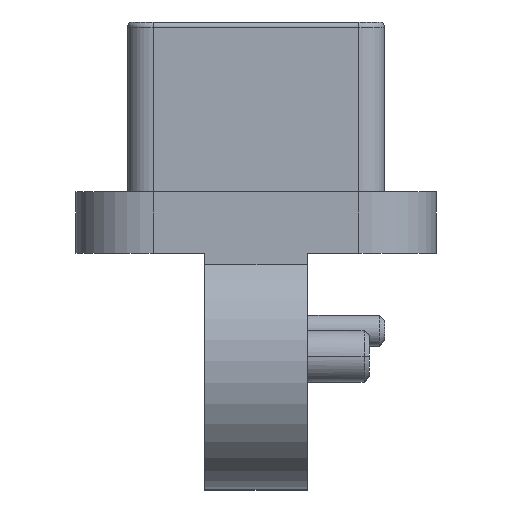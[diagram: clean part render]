
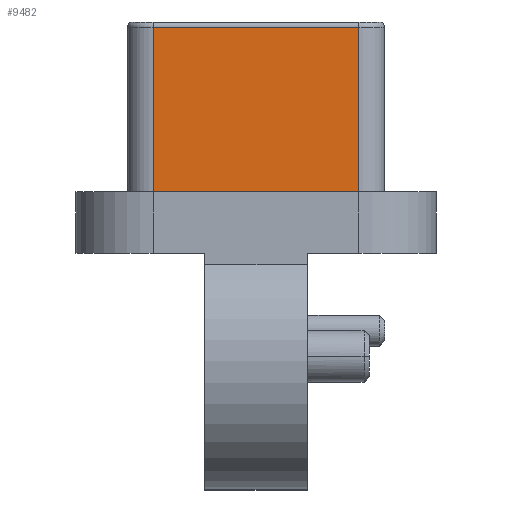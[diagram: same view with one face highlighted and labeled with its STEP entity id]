
A CAD part, left-side view. The second image highlights one B-rep face of the part: STEP entity #9482.
In plain terms, the highlighted planar face has unit normal (-1, 0, 0).
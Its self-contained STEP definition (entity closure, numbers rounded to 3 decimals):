
#28 = DIRECTION ( 'NONE',  ( 1., 0., 0. ) ) ;
#512 = CARTESIAN_POINT ( 'NONE',  ( -9.65, 2., -0.1 ) ) ;
#559 = CARTESIAN_POINT ( 'NONE',  ( -9.65, 2., -3.3 ) ) ;
#1010 = ORIENTED_EDGE ( 'NONE', *, *, #8530, .T. ) ;
#1637 = VERTEX_POINT ( 'NONE', #6849 ) ;
#2123 = CARTESIAN_POINT ( 'NONE',  ( -9.65, 0., -1.7 ) ) ;
#2163 = DIRECTION ( 'NONE',  ( 0., 0., 1. ) ) ;
#2252 = FACE_OUTER_BOUND ( 'NONE', #9941, .T. ) ;
#2441 = EDGE_CURVE ( 'NONE', #3061, #2565, #12146, .T. ) ;
#2565 = VERTEX_POINT ( 'NONE', #9912 ) ;
#2670 = VERTEX_POINT ( 'NONE', #6094 ) ;
#3061 = VERTEX_POINT ( 'NONE', #7101 ) ;
#3385 = LINE ( 'NONE', #6414, #11284 ) ;
#3459 = ORIENTED_EDGE ( 'NONE', *, *, #2441, .T. ) ;
#3780 = DIRECTION ( 'NONE',  ( 0., 0., -1. ) ) ;
#4279 = EDGE_CURVE ( 'NONE', #2670, #3061, #3385, .T. ) ;
#4369 = PLANE ( 'NONE',  #6392 ) ;
#4517 = DIRECTION ( 'NONE',  ( 0., 1., 0. ) ) ;
#4610 = VECTOR ( 'NONE', #2163, 1000. ) ;
#4827 = DIRECTION ( 'NONE',  ( 0., -1., 0. ) ) ;
#5419 = VECTOR ( 'NONE', #4827, 1000. ) ;
#5875 = LINE ( 'NONE', #559, #5419 ) ;
#6094 = CARTESIAN_POINT ( 'NONE',  ( -9.65, -2., -0.1 ) ) ;
#6103 = VECTOR ( 'NONE', #3780, 1000. ) ;
#6392 = AXIS2_PLACEMENT_3D ( 'NONE', #2123, #28, #11950 ) ;
#6414 = CARTESIAN_POINT ( 'NONE',  ( -9.65, -2., -0.1 ) ) ;
#6605 = CARTESIAN_POINT ( 'NONE',  ( -9.65, -2., -3.3 ) ) ;
#6849 = CARTESIAN_POINT ( 'NONE',  ( -9.65, -2., -3.3 ) ) ;
#7101 = CARTESIAN_POINT ( 'NONE',  ( -9.65, 2., -0.1 ) ) ;
#8005 = EDGE_CURVE ( 'NONE', #2565, #1637, #5875, .T. ) ;
#8046 = ORIENTED_EDGE ( 'NONE', *, *, #8005, .T. ) ;
#8530 = EDGE_CURVE ( 'NONE', #1637, #2670, #9774, .T. ) ;
#9482 = ADVANCED_FACE ( 'NONE', ( #2252 ), #4369, .F. ) ;
#9774 = LINE ( 'NONE', #6605, #4610 ) ;
#9912 = CARTESIAN_POINT ( 'NONE',  ( -9.65, 2., -3.3 ) ) ;
#9941 = EDGE_LOOP ( 'NONE', ( #3459, #8046, #1010, #12454 ) ) ;
#11284 = VECTOR ( 'NONE', #4517, 1000. ) ;
#11950 = DIRECTION ( 'NONE',  ( 0., 1., 0. ) ) ;
#12146 = LINE ( 'NONE', #512, #6103 ) ;
#12454 = ORIENTED_EDGE ( 'NONE', *, *, #4279, .T. ) ;
